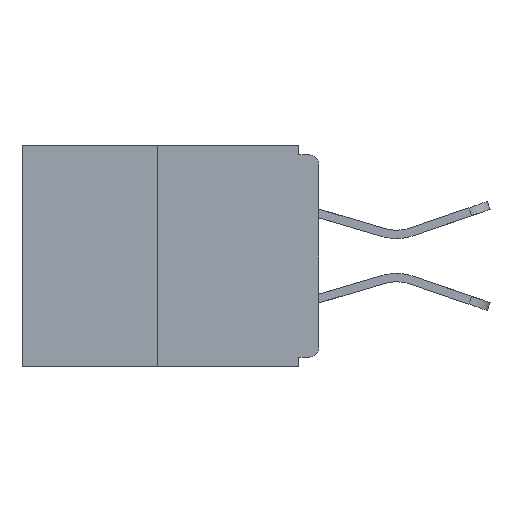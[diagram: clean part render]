
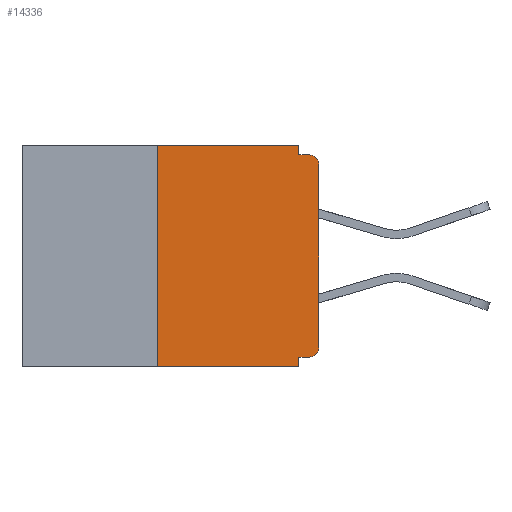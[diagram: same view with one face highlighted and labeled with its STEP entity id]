
A CAD part, left-side view. The second image highlights one B-rep face of the part: STEP entity #14336.
In plain terms, the highlighted planar face has unit normal (-1, 0, 0).
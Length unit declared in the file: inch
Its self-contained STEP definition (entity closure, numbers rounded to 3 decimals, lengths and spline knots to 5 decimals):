
#189 = ORIENTED_EDGE ( 'NONE', *, *, #14594, .T. ) ;
#190 = DIRECTION ( 'NONE',  ( -1., 0., 0. ) ) ;
#586 = ORIENTED_EDGE ( 'NONE', *, *, #1603, .F. ) ;
#707 = LINE ( 'NONE', #6180, #5488 ) ;
#860 = ORIENTED_EDGE ( 'NONE', *, *, #16894, .F. ) ;
#1309 = LINE ( 'NONE', #9391, #2023 ) ;
#1603 = EDGE_CURVE ( 'NONE', #12608, #11451, #5107, .T. ) ;
#1901 = CARTESIAN_POINT ( 'NONE',  ( 0., 0., -0.015 ) ) ;
#2014 = VECTOR ( 'NONE', #15202, 39.37008 ) ;
#2023 = VECTOR ( 'NONE', #16084, 39.37008 ) ;
#2062 = AXIS2_PLACEMENT_3D ( 'NONE', #13818, #8611, #2876 ) ;
#2152 = ORIENTED_EDGE ( 'NONE', *, *, #15901, .F. ) ;
#2876 = DIRECTION ( 'NONE',  ( 0., 0., -1. ) ) ;
#3141 = DIRECTION ( 'NONE',  ( 0., -1., 0. ) ) ;
#3259 = CIRCLE ( 'NONE', #10891, 0.015 ) ;
#3436 = DIRECTION ( 'NONE',  ( 0., 0., 1. ) ) ;
#3437 = VERTEX_POINT ( 'NONE', #9404 ) ;
#3730 = CARTESIAN_POINT ( 'NONE',  ( 0., 0.031, 0. ) ) ;
#3829 = CARTESIAN_POINT ( 'NONE',  ( 0., 0., 0. ) ) ;
#3872 = VERTEX_POINT ( 'NONE', #15989 ) ;
#5107 = LINE ( 'NONE', #14911, #12880 ) ;
#5132 = VERTEX_POINT ( 'NONE', #11184 ) ;
#5488 = VECTOR ( 'NONE', #13087, 39.37008 ) ;
#5491 = ORIENTED_EDGE ( 'NONE', *, *, #8407, .F. ) ;
#5977 = VERTEX_POINT ( 'NONE', #6446 ) ;
#6118 = VERTEX_POINT ( 'NONE', #15840 ) ;
#6180 = CARTESIAN_POINT ( 'NONE',  ( 0., 0.031, -0.343 ) ) ;
#6446 = CARTESIAN_POINT ( 'NONE',  ( 0., 0.031, -0.343 ) ) ;
#6708 = LINE ( 'NONE', #3829, #13230 ) ;
#7040 = ORIENTED_EDGE ( 'NONE', *, *, #13084, .T. ) ;
#7202 = DIRECTION ( 'NONE',  ( 0., 0., -1. ) ) ;
#7270 = LINE ( 'NONE', #1901, #9225 ) ;
#7317 = LINE ( 'NONE', #15729, #11169 ) ;
#7715 = VERTEX_POINT ( 'NONE', #17542 ) ;
#8099 = ORIENTED_EDGE ( 'NONE', *, *, #11222, .F. ) ;
#8407 = EDGE_CURVE ( 'NONE', #13845, #5132, #1309, .T. ) ;
#8488 = CARTESIAN_POINT ( 'NONE',  ( 0., 0.46, 0. ) ) ;
#8551 = DIRECTION ( 'NONE',  ( -1., 0., 0. ) ) ;
#8611 = DIRECTION ( 'NONE',  ( 1., 0., 0. ) ) ;
#8666 = EDGE_CURVE ( 'NONE', #7715, #17328, #11522, .T. ) ;
#9225 = VECTOR ( 'NONE', #3141, 39.37008 ) ;
#9391 = CARTESIAN_POINT ( 'NONE',  ( 0., 0.031, 0. ) ) ;
#9404 = CARTESIAN_POINT ( 'NONE',  ( 0., 0.015, -0.015 ) ) ;
#9696 = FACE_OUTER_BOUND ( 'NONE', #9856, .T. ) ;
#9856 = EDGE_LOOP ( 'NONE', ( #8099, #14764, #15758, #2152, #586, #7040, #189, #16948, #860, #5491 ) ) ;
#9873 = PLANE ( 'NONE',  #2062 ) ;
#10545 = DIRECTION ( 'NONE',  ( 0., 0., -1. ) ) ;
#10891 = AXIS2_PLACEMENT_3D ( 'NONE', #14676, #190, #10545 ) ;
#10960 = AXIS2_PLACEMENT_3D ( 'NONE', #15351, #8551, #7202 ) ;
#11169 = VECTOR ( 'NONE', #15546, 39.37008 ) ;
#11184 = CARTESIAN_POINT ( 'NONE',  ( 0., 0.031, -0.015 ) ) ;
#11222 = EDGE_CURVE ( 'NONE', #17328, #13845, #16452, .T. ) ;
#11451 = VERTEX_POINT ( 'NONE', #12865 ) ;
#11522 = LINE ( 'NONE', #11698, #14042 ) ;
#11698 = CARTESIAN_POINT ( 'NONE',  ( 0., 0.25, 0. ) ) ;
#11821 = CIRCLE ( 'NONE', #10960, 0.015 ) ;
#12004 = CARTESIAN_POINT ( 'NONE',  ( 0., 0.015, -0.328 ) ) ;
#12608 = VERTEX_POINT ( 'NONE', #12004 ) ;
#12865 = CARTESIAN_POINT ( 'NONE',  ( 0., 0.031, -0.328 ) ) ;
#12880 = VECTOR ( 'NONE', #16148, 39.37008 ) ;
#12944 = EDGE_CURVE ( 'NONE', #7715, #5977, #7317, .T. ) ;
#13084 = EDGE_CURVE ( 'NONE', #12608, #3872, #3259, .T. ) ;
#13087 = DIRECTION ( 'NONE',  ( 0., 0., -1. ) ) ;
#13230 = VECTOR ( 'NONE', #17627, 39.37008 ) ;
#13818 = CARTESIAN_POINT ( 'NONE',  ( 0., 0.46, 0. ) ) ;
#13845 = VERTEX_POINT ( 'NONE', #3730 ) ;
#14042 = VECTOR ( 'NONE', #3436, 39.37008 ) ;
#14336 = ADVANCED_FACE ( 'NONE', ( #9696 ), #9873, .F. ) ;
#14594 = EDGE_CURVE ( 'NONE', #3872, #6118, #6708, .T. ) ;
#14676 = CARTESIAN_POINT ( 'NONE',  ( 0., 0.015, -0.313 ) ) ;
#14764 = ORIENTED_EDGE ( 'NONE', *, *, #8666, .F. ) ;
#14911 = CARTESIAN_POINT ( 'NONE',  ( 0., 0., -0.328 ) ) ;
#15202 = DIRECTION ( 'NONE',  ( 0., -1., 0. ) ) ;
#15267 = EDGE_CURVE ( 'NONE', #6118, #3437, #11821, .T. ) ;
#15351 = CARTESIAN_POINT ( 'NONE',  ( 0., 0.015, -0.03 ) ) ;
#15390 = CARTESIAN_POINT ( 'NONE',  ( 0., 0.25, 0. ) ) ;
#15546 = DIRECTION ( 'NONE',  ( 0., -1., 0. ) ) ;
#15729 = CARTESIAN_POINT ( 'NONE',  ( 0., 0.46, -0.343 ) ) ;
#15758 = ORIENTED_EDGE ( 'NONE', *, *, #12944, .T. ) ;
#15840 = CARTESIAN_POINT ( 'NONE',  ( 0., 0., -0.03 ) ) ;
#15901 = EDGE_CURVE ( 'NONE', #11451, #5977, #707, .T. ) ;
#15989 = CARTESIAN_POINT ( 'NONE',  ( 0., 0., -0.313 ) ) ;
#16084 = DIRECTION ( 'NONE',  ( 0., 0., -1. ) ) ;
#16148 = DIRECTION ( 'NONE',  ( 0., 1., 0. ) ) ;
#16452 = LINE ( 'NONE', #8488, #2014 ) ;
#16894 = EDGE_CURVE ( 'NONE', #5132, #3437, #7270, .T. ) ;
#16948 = ORIENTED_EDGE ( 'NONE', *, *, #15267, .T. ) ;
#17328 = VERTEX_POINT ( 'NONE', #15390 ) ;
#17542 = CARTESIAN_POINT ( 'NONE',  ( 0., 0.25, -0.343 ) ) ;
#17627 = DIRECTION ( 'NONE',  ( 0., 0., 1. ) ) ;
